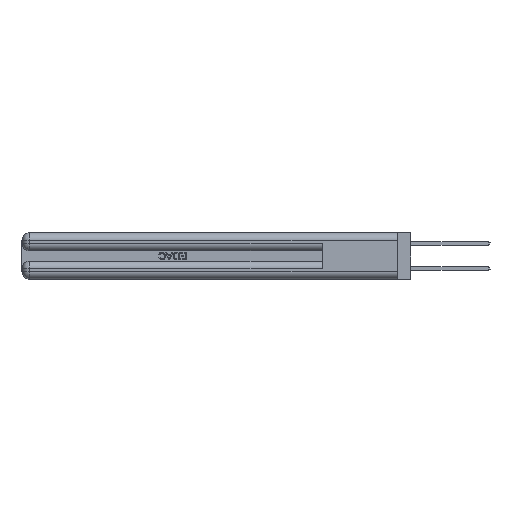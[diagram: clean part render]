
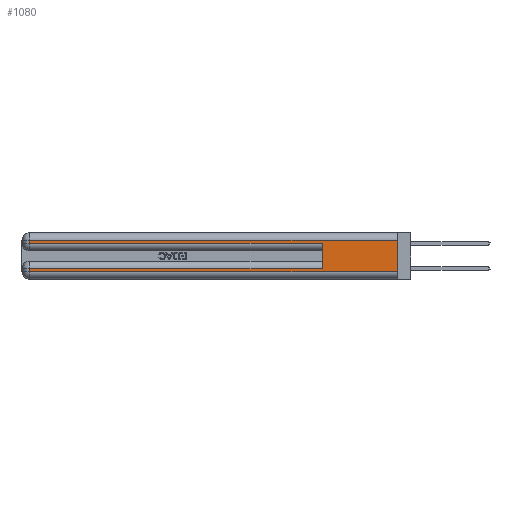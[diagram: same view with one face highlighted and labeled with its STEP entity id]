
A CAD part, left-side view. The second image highlights one B-rep face of the part: STEP entity #1080.
In plain terms, the highlighted planar face has unit normal (-1, 0, 0).
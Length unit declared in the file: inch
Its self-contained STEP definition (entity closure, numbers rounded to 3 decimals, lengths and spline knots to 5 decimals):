
#1080 = ADVANCED_FACE ( 'NONE', ( #11380 ), #30573, .F. ) ;
#1247 = LINE ( 'NONE', #23938, #40267 ) ;
#1652 = CARTESIAN_POINT ( 'NONE',  ( 0., 0., 0.285 ) ) ;
#4705 = VERTEX_POINT ( 'NONE', #22919 ) ;
#4941 = ORIENTED_EDGE ( 'NONE', *, *, #30022, .T. ) ;
#5787 = EDGE_CURVE ( 'NONE', #31151, #4705, #30016, .T. ) ;
#5998 = DIRECTION ( 'NONE',  ( 0., 0., -1. ) ) ;
#7518 = CARTESIAN_POINT ( 'NONE',  ( 0., 2.94, 0.31 ) ) ;
#7871 = LINE ( 'NONE', #23811, #44432 ) ;
#8079 = LINE ( 'NONE', #13756, #29195 ) ;
#8570 = LINE ( 'NONE', #1652, #26329 ) ;
#9378 = VECTOR ( 'NONE', #34098, 39.37008 ) ;
#10114 = LINE ( 'NONE', #36688, #27901 ) ;
#10195 = ORIENTED_EDGE ( 'NONE', *, *, #40332, .T. ) ;
#10890 = CARTESIAN_POINT ( 'NONE',  ( 0., 2.94, 0.085 ) ) ;
#11132 = VECTOR ( 'NONE', #43720, 39.37008 ) ;
#11380 = FACE_OUTER_BOUND ( 'NONE', #44458, .T. ) ;
#13756 = CARTESIAN_POINT ( 'NONE',  ( 0., 2.94, 0.37 ) ) ;
#14659 = AXIS2_PLACEMENT_3D ( 'NONE', #34108, #20042, #44748 ) ;
#15672 = DIRECTION ( 'NONE',  ( 0., 0., 1. ) ) ;
#17851 = EDGE_CURVE ( 'NONE', #43641, #4705, #7871, .T. ) ;
#18483 = CARTESIAN_POINT ( 'NONE',  ( 0., 0.6, 0.285 ) ) ;
#19002 = CARTESIAN_POINT ( 'NONE',  ( 0., 0., 0.06 ) ) ;
#19286 = EDGE_CURVE ( 'NONE', #38965, #42762, #43627, .T. ) ;
#20042 = DIRECTION ( 'NONE',  ( 1., 0., 0. ) ) ;
#21982 = EDGE_CURVE ( 'NONE', #38965, #45070, #10114, .T. ) ;
#22919 = CARTESIAN_POINT ( 'NONE',  ( 0., 0., 0.06 ) ) ;
#23607 = CARTESIAN_POINT ( 'NONE',  ( 0., 0., 0.31 ) ) ;
#23811 = CARTESIAN_POINT ( 'NONE',  ( 0., 0., 0.37 ) ) ;
#23938 = CARTESIAN_POINT ( 'NONE',  ( 0., 2.94, 0.37 ) ) ;
#24856 = VECTOR ( 'NONE', #34663, 39.37008 ) ;
#25182 = VERTEX_POINT ( 'NONE', #7518 ) ;
#26141 = EDGE_CURVE ( 'NONE', #43975, #45070, #8570, .T. ) ;
#26329 = VECTOR ( 'NONE', #37329, 39.37008 ) ;
#27901 = VECTOR ( 'NONE', #15672, 39.37008 ) ;
#29195 = VECTOR ( 'NONE', #31412, 39.37008 ) ;
#30016 = LINE ( 'NONE', #19002, #11132 ) ;
#30022 = EDGE_CURVE ( 'NONE', #43641, #25182, #30484, .T. ) ;
#30484 = LINE ( 'NONE', #23607, #9378 ) ;
#30573 = PLANE ( 'NONE',  #14659 ) ;
#30935 = DIRECTION ( 'NONE',  ( 0., 0., -1. ) ) ;
#31151 = VERTEX_POINT ( 'NONE', #37365 ) ;
#31412 = DIRECTION ( 'NONE',  ( 0., 0., -1. ) ) ;
#34098 = DIRECTION ( 'NONE',  ( 0., 1., 0. ) ) ;
#34108 = CARTESIAN_POINT ( 'NONE',  ( 0., 0., 0.37 ) ) ;
#34511 = CARTESIAN_POINT ( 'NONE',  ( 0., 0., 0.085 ) ) ;
#34663 = DIRECTION ( 'NONE',  ( 0., 1., 0. ) ) ;
#36208 = EDGE_CURVE ( 'NONE', #25182, #43975, #8079, .T. ) ;
#36361 = ORIENTED_EDGE ( 'NONE', *, *, #19286, .T. ) ;
#36688 = CARTESIAN_POINT ( 'NONE',  ( 0., 0.6, 0.145 ) ) ;
#37313 = ORIENTED_EDGE ( 'NONE', *, *, #21982, .F. ) ;
#37329 = DIRECTION ( 'NONE',  ( 0., -1., 0. ) ) ;
#37365 = CARTESIAN_POINT ( 'NONE',  ( 0., 2.94, 0.06 ) ) ;
#38965 = VERTEX_POINT ( 'NONE', #45185 ) ;
#39913 = CARTESIAN_POINT ( 'NONE',  ( 0., 0., 0.31 ) ) ;
#40267 = VECTOR ( 'NONE', #5998, 39.37008 ) ;
#40332 = EDGE_CURVE ( 'NONE', #42762, #31151, #1247, .T. ) ;
#41181 = ORIENTED_EDGE ( 'NONE', *, *, #36208, .T. ) ;
#41450 = CARTESIAN_POINT ( 'NONE',  ( 0., 2.94, 0.285 ) ) ;
#42762 = VERTEX_POINT ( 'NONE', #10890 ) ;
#43624 = ORIENTED_EDGE ( 'NONE', *, *, #17851, .F. ) ;
#43627 = LINE ( 'NONE', #34511, #24856 ) ;
#43641 = VERTEX_POINT ( 'NONE', #39913 ) ;
#43720 = DIRECTION ( 'NONE',  ( 0., -1., 0. ) ) ;
#43975 = VERTEX_POINT ( 'NONE', #41450 ) ;
#44432 = VECTOR ( 'NONE', #30935, 39.37008 ) ;
#44458 = EDGE_LOOP ( 'NONE', ( #43624, #4941, #41181, #45505, #37313, #36361, #10195, #45124 ) ) ;
#44748 = DIRECTION ( 'NONE',  ( 0., 0., -1. ) ) ;
#45070 = VERTEX_POINT ( 'NONE', #18483 ) ;
#45124 = ORIENTED_EDGE ( 'NONE', *, *, #5787, .T. ) ;
#45185 = CARTESIAN_POINT ( 'NONE',  ( 0., 0.6, 0.085 ) ) ;
#45505 = ORIENTED_EDGE ( 'NONE', *, *, #26141, .T. ) ;
